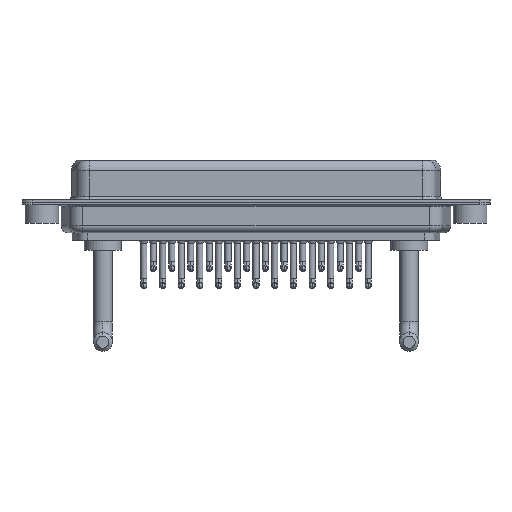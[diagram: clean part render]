
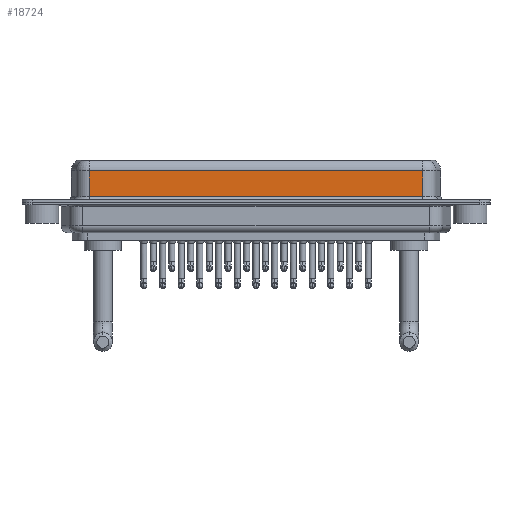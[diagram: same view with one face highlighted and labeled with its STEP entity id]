
A CAD part, front view. The second image highlights one B-rep face of the part: STEP entity #18724.
In plain terms, the highlighted planar face has unit normal (0, -1, 0).
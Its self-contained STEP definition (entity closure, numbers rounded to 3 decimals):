
#530 = LINE ( 'NONE', #4069, #9987 ) ;
#1668 = ORIENTED_EDGE ( 'NONE', *, *, #20447, .T. ) ;
#1794 = AXIS2_PLACEMENT_3D ( 'NONE', #24254, #3625, #12701 ) ;
#2894 = EDGE_CURVE ( 'NONE', #4949, #4241, #11329, .T. ) ;
#3346 = DIRECTION ( 'NONE',  ( 0., 0., -1. ) ) ;
#3625 = DIRECTION ( 'NONE',  ( 0., 1., 0. ) ) ;
#4069 = CARTESIAN_POINT ( 'NONE',  ( 56.462, -3.95, 0.9 ) ) ;
#4127 = CARTESIAN_POINT ( 'NONE',  ( 56.462, -3.95, 4.65 ) ) ;
#4241 = VERTEX_POINT ( 'NONE', #4895 ) ;
#4895 = CARTESIAN_POINT ( 'NONE',  ( 56.462, -3.95, 0.9 ) ) ;
#4949 = VERTEX_POINT ( 'NONE', #4127 ) ;
#6789 = VERTEX_POINT ( 'NONE', #15535 ) ;
#7153 = FACE_OUTER_BOUND ( 'NONE', #17178, .T. ) ;
#8843 = ORIENTED_EDGE ( 'NONE', *, *, #16035, .T. ) ;
#9279 = PLANE ( 'NONE',  #1794 ) ;
#9987 = VECTOR ( 'NONE', #16031, 1000. ) ;
#11199 = CARTESIAN_POINT ( 'NONE',  ( 56.462, -3.95, 6.4 ) ) ;
#11329 = LINE ( 'NONE', #11199, #15025 ) ;
#12701 = DIRECTION ( 'NONE',  ( 0., 0., 1. ) ) ;
#12858 = LINE ( 'NONE', #20035, #24018 ) ;
#14924 = CARTESIAN_POINT ( 'NONE',  ( 7.038, -3.95, 6.4 ) ) ;
#15025 = VECTOR ( 'NONE', #15116, 1000. ) ;
#15116 = DIRECTION ( 'NONE',  ( 0., 0., -1. ) ) ;
#15535 = CARTESIAN_POINT ( 'NONE',  ( 7.038, -3.95, 4.65 ) ) ;
#16031 = DIRECTION ( 'NONE',  ( 1., 0., 0. ) ) ;
#16035 = EDGE_CURVE ( 'NONE', #21361, #4241, #530, .T. ) ;
#16168 = ORIENTED_EDGE ( 'NONE', *, *, #22453, .T. ) ;
#16703 = ORIENTED_EDGE ( 'NONE', *, *, #2894, .F. ) ;
#17178 = EDGE_LOOP ( 'NONE', ( #16703, #16168, #1668, #8843 ) ) ;
#18638 = DIRECTION ( 'NONE',  ( -1., 0., 0. ) ) ;
#18724 = ADVANCED_FACE ( 'NONE', ( #7153 ), #9279, .F. ) ;
#20035 = CARTESIAN_POINT ( 'NONE',  ( 56.462, -3.95, 4.65 ) ) ;
#20206 = LINE ( 'NONE', #14924, #22783 ) ;
#20447 = EDGE_CURVE ( 'NONE', #6789, #21361, #20206, .T. ) ;
#21361 = VERTEX_POINT ( 'NONE', #23988 ) ;
#22453 = EDGE_CURVE ( 'NONE', #4949, #6789, #12858, .T. ) ;
#22783 = VECTOR ( 'NONE', #3346, 1000. ) ;
#23988 = CARTESIAN_POINT ( 'NONE',  ( 7.038, -3.95, 0.9 ) ) ;
#24018 = VECTOR ( 'NONE', #18638, 1000. ) ;
#24254 = CARTESIAN_POINT ( 'NONE',  ( 56.462, -3.95, 6.4 ) ) ;
